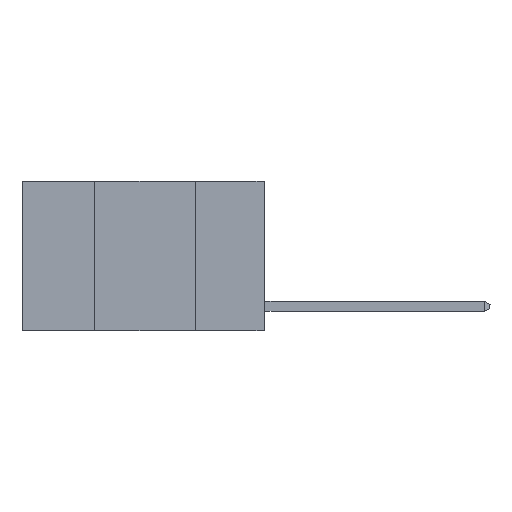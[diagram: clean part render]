
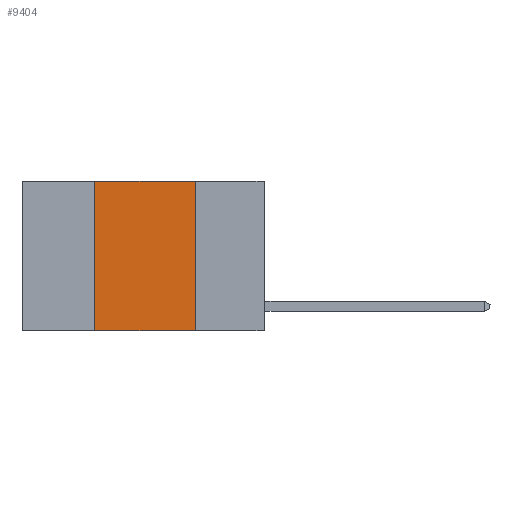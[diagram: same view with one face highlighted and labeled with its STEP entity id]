
A CAD part, left-side view. The second image highlights one B-rep face of the part: STEP entity #9404.
In plain terms, the highlighted planar face has unit normal (-1, 0, 0).
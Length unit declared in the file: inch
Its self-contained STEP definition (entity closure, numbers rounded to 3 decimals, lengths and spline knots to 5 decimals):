
#22 = EDGE_CURVE ( 'NONE', #1181, #8414, #6135, .T. ) ;
#48 = VECTOR ( 'NONE', #4178, 39.37008 ) ;
#291 = VERTEX_POINT ( 'NONE', #3953 ) ;
#427 = VECTOR ( 'NONE', #7408, 39.37008 ) ;
#922 = DIRECTION ( 'NONE',  ( 0., 0., -1. ) ) ;
#1181 = VERTEX_POINT ( 'NONE', #11403 ) ;
#2334 = CARTESIAN_POINT ( 'NONE',  ( 0., 0.6, -0.37 ) ) ;
#2500 = AXIS2_PLACEMENT_3D ( 'NONE', #12442, #12490, #922 ) ;
#2575 = EDGE_CURVE ( 'NONE', #11724, #291, #5531, .T. ) ;
#2838 = LINE ( 'NONE', #12213, #48 ) ;
#2930 = PLANE ( 'NONE',  #2500 ) ;
#3400 = VECTOR ( 'NONE', #4031, 39.37008 ) ;
#3651 = CARTESIAN_POINT ( 'NONE',  ( 0., 0.17, 0. ) ) ;
#3953 = CARTESIAN_POINT ( 'NONE',  ( 0., 0.17, -0.37 ) ) ;
#4031 = DIRECTION ( 'NONE',  ( 0., 0., 1. ) ) ;
#4178 = DIRECTION ( 'NONE',  ( 0., 0., -1. ) ) ;
#4970 = EDGE_CURVE ( 'NONE', #11724, #1181, #13569, .T. ) ;
#5145 = CARTESIAN_POINT ( 'NONE',  ( 0., 0.42, 0. ) ) ;
#5531 = LINE ( 'NONE', #2334, #427 ) ;
#5679 = VECTOR ( 'NONE', #11493, 39.37008 ) ;
#5923 = ORIENTED_EDGE ( 'NONE', *, *, #4970, .F. ) ;
#6135 = LINE ( 'NONE', #8356, #5679 ) ;
#6777 = ORIENTED_EDGE ( 'NONE', *, *, #22, .F. ) ;
#6959 = ORIENTED_EDGE ( 'NONE', *, *, #10953, .F. ) ;
#7408 = DIRECTION ( 'NONE',  ( 0., -1., 0. ) ) ;
#8356 = CARTESIAN_POINT ( 'NONE',  ( 0., 0.6, 0. ) ) ;
#8414 = VERTEX_POINT ( 'NONE', #3651 ) ;
#8858 = CARTESIAN_POINT ( 'NONE',  ( 0., 0.42, -0.37 ) ) ;
#9259 = ORIENTED_EDGE ( 'NONE', *, *, #2575, .T. ) ;
#9404 = ADVANCED_FACE ( 'NONE', ( #12931 ), #2930, .F. ) ;
#9749 = EDGE_LOOP ( 'NONE', ( #6959, #6777, #5923, #9259 ) ) ;
#10953 = EDGE_CURVE ( 'NONE', #8414, #291, #2838, .T. ) ;
#11403 = CARTESIAN_POINT ( 'NONE',  ( 0., 0.42, 0. ) ) ;
#11493 = DIRECTION ( 'NONE',  ( 0., -1., 0. ) ) ;
#11724 = VERTEX_POINT ( 'NONE', #8858 ) ;
#12213 = CARTESIAN_POINT ( 'NONE',  ( 0., 0.17, 0. ) ) ;
#12442 = CARTESIAN_POINT ( 'NONE',  ( 0., 0.6, 0. ) ) ;
#12490 = DIRECTION ( 'NONE',  ( 1., 0., 0. ) ) ;
#12931 = FACE_OUTER_BOUND ( 'NONE', #9749, .T. ) ;
#13569 = LINE ( 'NONE', #5145, #3400 ) ;
